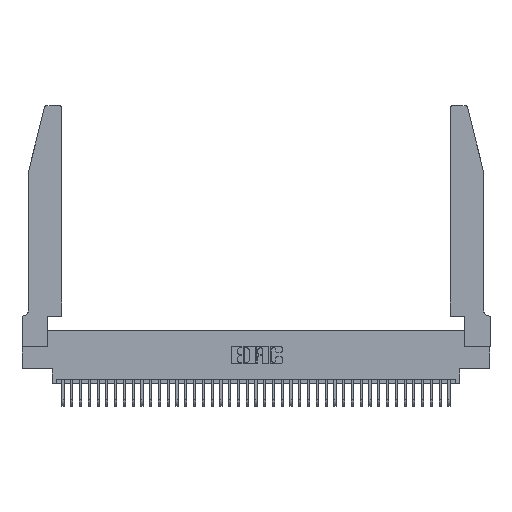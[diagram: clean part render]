
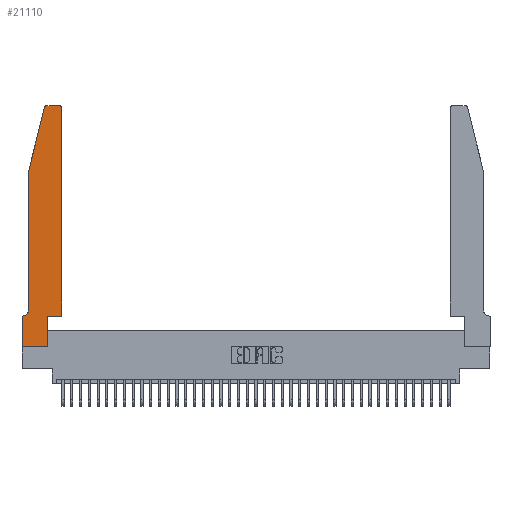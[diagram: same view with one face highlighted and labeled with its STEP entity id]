
A CAD part, top view. The second image highlights one B-rep face of the part: STEP entity #21110.
In plain terms, the highlighted planar face has unit normal (0, 0, 1).
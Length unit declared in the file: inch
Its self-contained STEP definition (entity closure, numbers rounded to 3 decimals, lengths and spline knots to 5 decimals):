
#8 = ORIENTED_EDGE ( 'NONE', *, *, #11257, .T. ) ;
#330 = VERTEX_POINT ( 'NONE', #36066 ) ;
#732 = LINE ( 'NONE', #9962, #1677 ) ;
#1677 = VECTOR ( 'NONE', #30722, 39.37008 ) ;
#1902 = VERTEX_POINT ( 'NONE', #37615 ) ;
#2230 = CARTESIAN_POINT ( 'NONE',  ( 0.0755, 0.35, 0.37 ) ) ;
#2847 = CARTESIAN_POINT ( 'NONE',  ( 0., 0., 0.37 ) ) ;
#3303 = LINE ( 'NONE', #8295, #25117 ) ;
#3494 = VERTEX_POINT ( 'NONE', #30942 ) ;
#3583 = VERTEX_POINT ( 'NONE', #16555 ) ;
#3628 = CARTESIAN_POINT ( 'NONE',  ( 0.4505, 0.35, 0.37 ) ) ;
#4030 = EDGE_CURVE ( 'NONE', #33637, #3494, #13621, .T. ) ;
#4116 = EDGE_CURVE ( 'NONE', #1902, #7216, #31678, .T. ) ;
#4514 = ORIENTED_EDGE ( 'NONE', *, *, #5517, .T. ) ;
#4549 = CARTESIAN_POINT ( 'NONE',  ( 0.0755, 2., 0.37 ) ) ;
#5404 = LINE ( 'NONE', #32359, #35979 ) ;
#5517 = EDGE_CURVE ( 'NONE', #330, #34089, #9752, .T. ) ;
#5563 = ORIENTED_EDGE ( 'NONE', *, *, #22402, .T. ) ;
#5633 = CARTESIAN_POINT ( 'NONE',  ( 0.4205, 2.75, 0.37 ) ) ;
#5985 = AXIS2_PLACEMENT_3D ( 'NONE', #29185, #11448, #32163 ) ;
#6481 = EDGE_CURVE ( 'NONE', #3494, #330, #22671, .T. ) ;
#6869 = CARTESIAN_POINT ( 'NONE',  ( 0.0755, 0.42, 0.37 ) ) ;
#7216 = VERTEX_POINT ( 'NONE', #19459 ) ;
#7467 = VERTEX_POINT ( 'NONE', #20607 ) ;
#7690 = DIRECTION ( 'NONE',  ( -0.239, -0.971, 0. ) ) ;
#7713 = EDGE_CURVE ( 'NONE', #34310, #3583, #732, .T. ) ;
#7876 = DIRECTION ( 'NONE',  ( 0., 0., -1. ) ) ;
#7901 = VERTEX_POINT ( 'NONE', #38403 ) ;
#8295 = CARTESIAN_POINT ( 'NONE',  ( 0.4505, 0.35, 0.37 ) ) ;
#8810 = EDGE_CURVE ( 'NONE', #7216, #15885, #18355, .T. ) ;
#8836 = VECTOR ( 'NONE', #7690, 39.37008 ) ;
#9553 = VECTOR ( 'NONE', #31397, 39.37008 ) ;
#9752 = LINE ( 'NONE', #16510, #8836 ) ;
#9962 = CARTESIAN_POINT ( 'NONE',  ( 0.2865, 0.35, 0.37 ) ) ;
#10795 = EDGE_CURVE ( 'NONE', #3583, #7467, #36024, .T. ) ;
#11257 = EDGE_CURVE ( 'NONE', #15885, #34310, #5404, .T. ) ;
#11448 = DIRECTION ( 'NONE',  ( 0., 0., 1. ) ) ;
#12663 = VECTOR ( 'NONE', #28289, 39.37008 ) ;
#13128 = DIRECTION ( 'NONE',  ( 0., 0., 1. ) ) ;
#13587 = FACE_OUTER_BOUND ( 'NONE', #26790, .T. ) ;
#13621 = LINE ( 'NONE', #34131, #12663 ) ;
#13669 = CARTESIAN_POINT ( 'NONE',  ( 0., 0., 0.37 ) ) ;
#14398 = CARTESIAN_POINT ( 'NONE',  ( 0.2865, 0., 0.37 ) ) ;
#15048 = ORIENTED_EDGE ( 'NONE', *, *, #4116, .T. ) ;
#15651 = DIRECTION ( 'NONE',  ( 0., 0., 1. ) ) ;
#15885 = VERTEX_POINT ( 'NONE', #2847 ) ;
#16510 = CARTESIAN_POINT ( 'NONE',  ( 0.0755, 2., 0.37 ) ) ;
#16555 = CARTESIAN_POINT ( 'NONE',  ( 0.2865, 0.35, 0.37 ) ) ;
#17604 = DIRECTION ( 'NONE',  ( 1., 0., 0. ) ) ;
#18355 = LINE ( 'NONE', #13669, #9553 ) ;
#18735 = AXIS2_PLACEMENT_3D ( 'NONE', #24948, #13128, #33845 ) ;
#18825 = VERTEX_POINT ( 'NONE', #6869 ) ;
#18960 = ORIENTED_EDGE ( 'NONE', *, *, #26791, .T. ) ;
#19459 = CARTESIAN_POINT ( 'NONE',  ( 0., 0.35, 0.37 ) ) ;
#20607 = CARTESIAN_POINT ( 'NONE',  ( 0.4505, 0.35, 0.37 ) ) ;
#21110 = ADVANCED_FACE ( 'NONE', ( #13587 ), #36686, .T. ) ;
#21358 = DIRECTION ( 'NONE',  ( 1., 0., 0. ) ) ;
#22402 = EDGE_CURVE ( 'NONE', #18825, #1902, #35136, .T. ) ;
#22671 = CIRCLE ( 'NONE', #36171, 0.03 ) ;
#23796 = VECTOR ( 'NONE', #28951, 39.37008 ) ;
#23843 = CARTESIAN_POINT ( 'NONE',  ( 0.0755, 2., 0.37 ) ) ;
#24948 = CARTESIAN_POINT ( 'NONE',  ( 0., 0.35, 0.37 ) ) ;
#25117 = VECTOR ( 'NONE', #28881, 39.37008 ) ;
#25635 = CARTESIAN_POINT ( 'NONE',  ( 0.0055, 0.42, 0.37 ) ) ;
#26790 = EDGE_LOOP ( 'NONE', ( #27472, #35597, #4514, #29020, #5563, #15048, #32422, #8, #32203, #31461, #18960, #37141 ) ) ;
#26791 = EDGE_CURVE ( 'NONE', #7467, #7901, #3303, .T. ) ;
#27472 = ORIENTED_EDGE ( 'NONE', *, *, #4030, .T. ) ;
#27698 = CIRCLE ( 'NONE', #5985, 0.03 ) ;
#27988 = VECTOR ( 'NONE', #29794, 39.37008 ) ;
#28148 = VECTOR ( 'NONE', #21358, 39.37008 ) ;
#28289 = DIRECTION ( 'NONE',  ( -1., 0., 0. ) ) ;
#28441 = AXIS2_PLACEMENT_3D ( 'NONE', #25635, #7876, #28599 ) ;
#28599 = DIRECTION ( 'NONE',  ( -1., 0., 0. ) ) ;
#28881 = DIRECTION ( 'NONE',  ( 0., 1., 0. ) ) ;
#28951 = DIRECTION ( 'NONE',  ( -1., 0., 0. ) ) ;
#29020 = ORIENTED_EDGE ( 'NONE', *, *, #38353, .T. ) ;
#29185 = CARTESIAN_POINT ( 'NONE',  ( 0.4205, 2.72, 0.37 ) ) ;
#29794 = DIRECTION ( 'NONE',  ( 0., -1., 0. ) ) ;
#30722 = DIRECTION ( 'NONE',  ( 0., 1., 0. ) ) ;
#30942 = CARTESIAN_POINT ( 'NONE',  ( 0.284, 2.75, 0.37 ) ) ;
#31397 = DIRECTION ( 'NONE',  ( 0., -1., 0. ) ) ;
#31461 = ORIENTED_EDGE ( 'NONE', *, *, #10795, .T. ) ;
#31678 = LINE ( 'NONE', #2230, #23796 ) ;
#32163 = DIRECTION ( 'NONE',  ( 1., 0., 0. ) ) ;
#32203 = ORIENTED_EDGE ( 'NONE', *, *, #7713, .T. ) ;
#32359 = CARTESIAN_POINT ( 'NONE',  ( 0., 0., 0.37 ) ) ;
#32422 = ORIENTED_EDGE ( 'NONE', *, *, #8810, .T. ) ;
#33380 = CARTESIAN_POINT ( 'NONE',  ( 0.284, 2.72, 0.37 ) ) ;
#33637 = VERTEX_POINT ( 'NONE', #5633 ) ;
#33845 = DIRECTION ( 'NONE',  ( 1., 0., 0. ) ) ;
#34089 = VERTEX_POINT ( 'NONE', #4549 ) ;
#34131 = CARTESIAN_POINT ( 'NONE',  ( 0.2605, 2.75, 0.37 ) ) ;
#34310 = VERTEX_POINT ( 'NONE', #14398 ) ;
#35136 = CIRCLE ( 'NONE', #28441, 0.07 ) ;
#35597 = ORIENTED_EDGE ( 'NONE', *, *, #6481, .T. ) ;
#35859 = LINE ( 'NONE', #23843, #27988 ) ;
#35979 = VECTOR ( 'NONE', #17604, 39.37008 ) ;
#36024 = LINE ( 'NONE', #3628, #28148 ) ;
#36066 = CARTESIAN_POINT ( 'NONE',  ( 0.25487, 2.72718, 0.37 ) ) ;
#36171 = AXIS2_PLACEMENT_3D ( 'NONE', #33380, #15651, #36355 ) ;
#36353 = EDGE_CURVE ( 'NONE', #7901, #33637, #27698, .T. ) ;
#36355 = DIRECTION ( 'NONE',  ( 1., 0., 0. ) ) ;
#36686 = PLANE ( 'NONE',  #18735 ) ;
#37141 = ORIENTED_EDGE ( 'NONE', *, *, #36353, .T. ) ;
#37615 = CARTESIAN_POINT ( 'NONE',  ( 0.0055, 0.35, 0.37 ) ) ;
#38353 = EDGE_CURVE ( 'NONE', #34089, #18825, #35859, .T. ) ;
#38403 = CARTESIAN_POINT ( 'NONE',  ( 0.4505, 2.72, 0.37 ) ) ;
